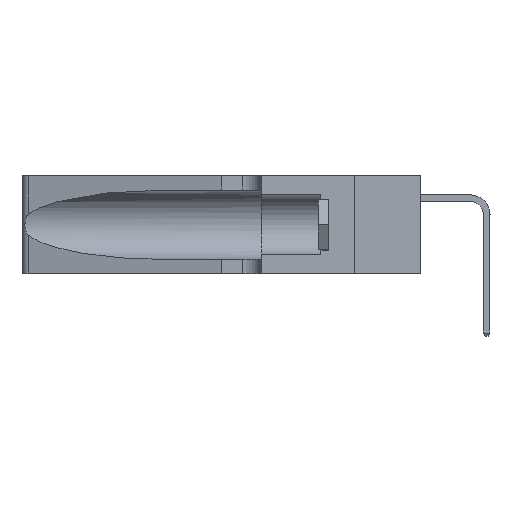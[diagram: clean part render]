
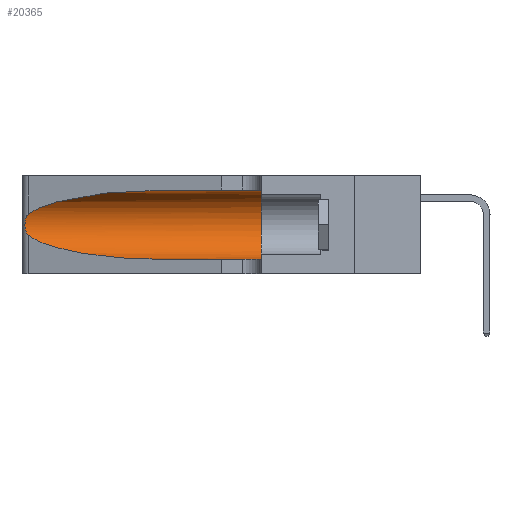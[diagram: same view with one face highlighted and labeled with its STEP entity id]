
A CAD part, left-side view. The second image highlights one B-rep face of the part: STEP entity #20365.
In plain terms, the highlighted cylindrical face has radius 3.308 mm (diameter 6.617 mm), a partial arc.
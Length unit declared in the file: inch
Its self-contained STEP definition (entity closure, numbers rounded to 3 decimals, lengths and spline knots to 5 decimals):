
#175 = CARTESIAN_POINT ( 'NONE',  ( 0.18966, 0.96281, 0.31525 ) ) ;
#427 = LINE ( 'NONE', #1715, #8719 ) ;
#652 = CARTESIAN_POINT ( 'NONE',  ( 0.1305, 0.72297, 0.05475 ) ) ;
#691 = FACE_OUTER_BOUND ( 'NONE', #3147, .T. ) ;
#758 = CARTESIAN_POINT ( 'NONE',  ( 0.25555, 1.22994, 0.2215 ) ) ;
#831 = CARTESIAN_POINT ( 'NONE',  ( 0.25555, 1.22993, 0.14849 ) ) ;
#991 = DIRECTION ( 'NONE',  ( 0., 0., -1. ) ) ;
#1132 = DIRECTION ( 'NONE',  ( 0., -1., 0. ) ) ;
#1505 =( BOUNDED_CURVE ( )  B_SPLINE_CURVE ( 3, ( #10425, #3971, #10495, #652 ),
 .UNSPECIFIED., .F., .T. ) 
 B_SPLINE_CURVE_WITH_KNOTS ( ( 4, 4 ),
 ( 3.44316, 4.71239 ),
 .UNSPECIFIED. ) 
 CURVE ( )  GEOMETRIC_REPRESENTATION_ITEM ( )  RATIONAL_B_SPLINE_CURVE ( ( 1., 0.87, 0.87, 1. ) ) 
 REPRESENTATION_ITEM ( '' )  );
#1702 = ORIENTED_EDGE ( 'NONE', *, *, #1944, .F. ) ;
#1715 = CARTESIAN_POINT ( 'NONE',  ( 0.1305, 1.61858, 0.31525 ) ) ;
#1800 = CARTESIAN_POINT ( 'NONE',  ( 0.1305, 0.35, 0.05475 ) ) ;
#1841 = CARTESIAN_POINT ( 'NONE',  ( 0.2373, 1.15595, 0.28018 ) ) ;
#1944 = EDGE_CURVE ( 'NONE', #13011, #16142, #15969, .T. ) ;
#2010 = VERTEX_POINT ( 'NONE', #4541 ) ;
#2712 = CARTESIAN_POINT ( 'NONE',  ( 0.25487, 1.22718, 0.22369 ) ) ;
#3147 = EDGE_LOOP ( 'NONE', ( #14695, #9818, #11863, #15246, #1702, #5580 ) ) ;
#3925 = EDGE_CURVE ( 'NONE', #10550, #16142, #11888, .T. ) ;
#3971 = CARTESIAN_POINT ( 'NONE',  ( 0.2373, 1.15595, 0.08982 ) ) ;
#4138 = CARTESIAN_POINT ( 'NONE',  ( 0.25787, 1.23484, 0.2124 ) ) ;
#4541 = CARTESIAN_POINT ( 'NONE',  ( 0.25487, 1.22718, 0.14631 ) ) ;
#5580 = ORIENTED_EDGE ( 'NONE', *, *, #20549, .F. ) ;
#5842 = CARTESIAN_POINT ( 'NONE',  ( 0.26018, 1.23835, 0.19895 ) ) ;
#6372 = VERTEX_POINT ( 'NONE', #10999 ) ;
#6829 = EDGE_CURVE ( 'NONE', #2010, #10550, #1505, .T. ) ;
#7455 = CARTESIAN_POINT ( 'NONE',  ( 0.26075, 1.23896, 0.178 ) ) ;
#8719 = VECTOR ( 'NONE', #14697, 39.37008 ) ;
#8753 = VERTEX_POINT ( 'NONE', #2712 ) ;
#9083 = CARTESIAN_POINT ( 'NONE',  ( 0.25856, 1.23593, 0.16098 ) ) ;
#9818 = ORIENTED_EDGE ( 'NONE', *, *, #14555, .T. ) ;
#9954 =( BOUNDED_CURVE ( )  B_SPLINE_CURVE ( 3, ( #10031, #175, #1841, #13230 ),
 .UNSPECIFIED., .F., .F. ) 
 B_SPLINE_CURVE_WITH_KNOTS ( ( 4, 4 ),
 ( 1.5708, 2.84003 ),
 .UNSPECIFIED. ) 
 CURVE ( )  GEOMETRIC_REPRESENTATION_ITEM ( )  RATIONAL_B_SPLINE_CURVE ( ( 1., 0.87, 0.87, 1. ) ) 
 REPRESENTATION_ITEM ( '' )  );
#10031 = CARTESIAN_POINT ( 'NONE',  ( 0.1305, 0.72297, 0.31525 ) ) ;
#10243 = CARTESIAN_POINT ( 'NONE',  ( 0.1305, 0.35, 0.185 ) ) ;
#10425 = CARTESIAN_POINT ( 'NONE',  ( 0.25487, 1.22718, 0.14631 ) ) ;
#10495 = CARTESIAN_POINT ( 'NONE',  ( 0.18966, 0.96281, 0.05475 ) ) ;
#10550 = VERTEX_POINT ( 'NONE', #13270 ) ;
#10657 = CARTESIAN_POINT ( 'NONE',  ( 0.25639, 1.23186, 0.15144 ) ) ;
#10870 = CARTESIAN_POINT ( 'NONE',  ( 0.1305, 1.61858, 0.185 ) ) ;
#10999 = CARTESIAN_POINT ( 'NONE',  ( 0.1305, 0.72297, 0.31525 ) ) ;
#11119 = AXIS2_PLACEMENT_3D ( 'NONE', #10870, #1132, #991 ) ;
#11130 = AXIS2_PLACEMENT_3D ( 'NONE', #10243, #12036, #12311 ) ;
#11863 = ORIENTED_EDGE ( 'NONE', *, *, #6829, .T. ) ;
#11888 = LINE ( 'NONE', #16435, #13891 ) ;
#12036 = DIRECTION ( 'NONE',  ( 0., 1., 0. ) ) ;
#12186 = CARTESIAN_POINT ( 'NONE',  ( 0.25487, 1.22718, 0.22369 ) ) ;
#12191 = CYLINDRICAL_SURFACE ( 'NONE', #11119, 0.13025 ) ;
#12254 = CARTESIAN_POINT ( 'NONE',  ( 0.25487, 1.22718, 0.14631 ) ) ;
#12311 = DIRECTION ( 'NONE',  ( 0., 0., 1. ) ) ;
#13011 = VERTEX_POINT ( 'NONE', #17774 ) ;
#13230 = CARTESIAN_POINT ( 'NONE',  ( 0.25487, 1.22718, 0.22369 ) ) ;
#13270 = CARTESIAN_POINT ( 'NONE',  ( 0.1305, 0.72297, 0.05475 ) ) ;
#13391 = DIRECTION ( 'NONE',  ( 0., -1., 0. ) ) ;
#13783 = CARTESIAN_POINT ( 'NONE',  ( 0.25639, 1.23184, 0.21858 ) ) ;
#13891 = VECTOR ( 'NONE', #13391, 39.37008 ) ;
#14555 = EDGE_CURVE ( 'NONE', #8753, #2010, #20110, .T. ) ;
#14695 = ORIENTED_EDGE ( 'NONE', *, *, #16826, .T. ) ;
#14697 = DIRECTION ( 'NONE',  ( 0., -1., 0. ) ) ;
#15246 = ORIENTED_EDGE ( 'NONE', *, *, #3925, .T. ) ;
#15381 = CARTESIAN_POINT ( 'NONE',  ( 0.25854, 1.2359, 0.20912 ) ) ;
#15969 = CIRCLE ( 'NONE', #11130, 0.13025 ) ;
#16142 = VERTEX_POINT ( 'NONE', #1800 ) ;
#16435 = CARTESIAN_POINT ( 'NONE',  ( 0.1305, 1.61858, 0.05475 ) ) ;
#16826 = EDGE_CURVE ( 'NONE', #6372, #8753, #9954, .T. ) ;
#16976 = CARTESIAN_POINT ( 'NONE',  ( 0.26075, 1.23896, 0.19203 ) ) ;
#17774 = CARTESIAN_POINT ( 'NONE',  ( 0.1305, 0.35, 0.31525 ) ) ;
#18571 = CARTESIAN_POINT ( 'NONE',  ( 0.26017, 1.23833, 0.17102 ) ) ;
#20110 = B_SPLINE_CURVE_WITH_KNOTS ( 'NONE', 3,
 ( #12186, #758, #13783, #4138, #15381, #5842, #16976, #7455, #18571, #9083, #20147, #10657, #831, #12254 ),
 .UNSPECIFIED., .F., .F.,
 ( 4, 2, 2, 2, 2, 2, 4 ),
 ( 0., 0.00027, 0.00053, 0.00107, 0.0016, 0.00187, 0.00214 ),
 .UNSPECIFIED. ) ;
#20147 = CARTESIAN_POINT ( 'NONE',  ( 0.25789, 1.23486, 0.15765 ) ) ;
#20365 = ADVANCED_FACE ( 'NONE', ( #691 ), #12191, .F. ) ;
#20549 = EDGE_CURVE ( 'NONE', #6372, #13011, #427, .T. ) ;
